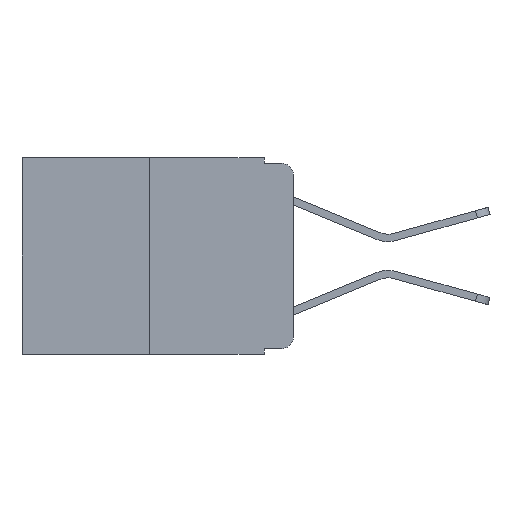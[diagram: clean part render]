
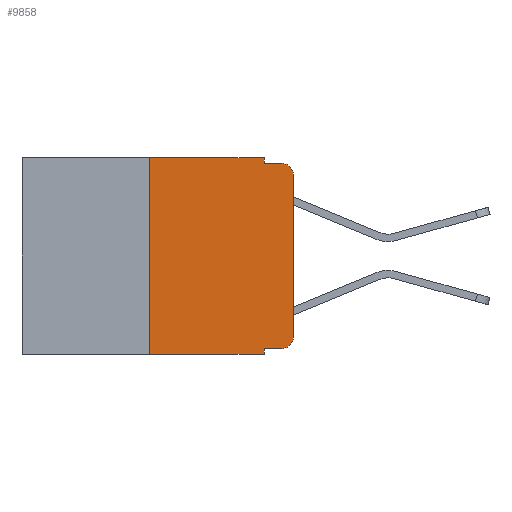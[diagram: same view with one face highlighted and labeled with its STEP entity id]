
A CAD part, left-side view. The second image highlights one B-rep face of the part: STEP entity #9858.
In plain terms, the highlighted planar face has unit normal (-1, 0, 0).
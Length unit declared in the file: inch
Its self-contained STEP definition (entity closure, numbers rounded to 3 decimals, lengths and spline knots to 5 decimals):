
#457 = CARTESIAN_POINT ( 'NONE',  ( 0., 0.25, 0. ) ) ;
#943 = EDGE_CURVE ( 'NONE', #7155, #8708, #5333, .T. ) ;
#949 = CARTESIAN_POINT ( 'NONE',  ( 0., 0.051, -0.333 ) ) ;
#1145 = ORIENTED_EDGE ( 'NONE', *, *, #11439, .T. ) ;
#1401 = DIRECTION ( 'NONE',  ( 0., 0., -1. ) ) ;
#1441 = ORIENTED_EDGE ( 'NONE', *, *, #943, .F. ) ;
#1490 = DIRECTION ( 'NONE',  ( 0., 0., 1. ) ) ;
#1531 = CARTESIAN_POINT ( 'NONE',  ( 0., 0.051, -0.333 ) ) ;
#1535 = PLANE ( 'NONE',  #4030 ) ;
#1721 = ORIENTED_EDGE ( 'NONE', *, *, #6857, .T. ) ;
#1846 = EDGE_CURVE ( 'NONE', #9617, #7839, #5854, .T. ) ;
#1906 = VECTOR ( 'NONE', #2562, 39.37008 ) ;
#1918 = CARTESIAN_POINT ( 'NONE',  ( 0., 0.02, -0.03 ) ) ;
#1947 = ORIENTED_EDGE ( 'NONE', *, *, #4604, .T. ) ;
#2239 = ORIENTED_EDGE ( 'NONE', *, *, #6475, .T. ) ;
#2348 = ORIENTED_EDGE ( 'NONE', *, *, #1846, .F. ) ;
#2426 = ORIENTED_EDGE ( 'NONE', *, *, #5461, .T. ) ;
#2505 = CARTESIAN_POINT ( 'NONE',  ( 0., 0.02, -0.313 ) ) ;
#2562 = DIRECTION ( 'NONE',  ( 0., -1., 0. ) ) ;
#2704 = VECTOR ( 'NONE', #1490, 39.37008 ) ;
#2751 = ORIENTED_EDGE ( 'NONE', *, *, #11470, .F. ) ;
#2771 = EDGE_CURVE ( 'NONE', #4984, #7155, #8645, .T. ) ;
#2778 = ORIENTED_EDGE ( 'NONE', *, *, #10975, .F. ) ;
#2969 = DIRECTION ( 'NONE',  ( 0., 0., -1. ) ) ;
#3091 = CARTESIAN_POINT ( 'NONE',  ( 0., 0.051, -0.01 ) ) ;
#3151 = CARTESIAN_POINT ( 'NONE',  ( 0., 0., -0.03 ) ) ;
#3328 = ORIENTED_EDGE ( 'NONE', *, *, #2771, .F. ) ;
#3361 = VECTOR ( 'NONE', #6061, 39.37008 ) ;
#3506 = CARTESIAN_POINT ( 'NONE',  ( 0., 0., 0. ) ) ;
#3539 = DIRECTION ( 'NONE',  ( 0., 0., -1. ) ) ;
#3949 = CARTESIAN_POINT ( 'NONE',  ( 0., 0.02, -0.333 ) ) ;
#4030 = AXIS2_PLACEMENT_3D ( 'NONE', #5511, #12036, #6426 ) ;
#4118 = DIRECTION ( 'NONE',  ( 0., -1., 0. ) ) ;
#4193 = VERTEX_POINT ( 'NONE', #4708 ) ;
#4548 = LINE ( 'NONE', #7319, #1906 ) ;
#4604 = EDGE_CURVE ( 'NONE', #4193, #6598, #8902, .T. ) ;
#4708 = CARTESIAN_POINT ( 'NONE',  ( 0., 0., -0.313 ) ) ;
#4772 = VERTEX_POINT ( 'NONE', #8410 ) ;
#4984 = VERTEX_POINT ( 'NONE', #6372 ) ;
#5025 = LINE ( 'NONE', #1531, #12170 ) ;
#5037 = VECTOR ( 'NONE', #8618, 39.37008 ) ;
#5267 = CIRCLE ( 'NONE', #10275, 0.02 ) ;
#5333 = LINE ( 'NONE', #7799, #5037 ) ;
#5461 = EDGE_CURVE ( 'NONE', #7344, #7839, #9170, .T. ) ;
#5469 = DIRECTION ( 'NONE',  ( 0., 0., 1. ) ) ;
#5511 = CARTESIAN_POINT ( 'NONE',  ( 0., 0.473, 0. ) ) ;
#5854 = LINE ( 'NONE', #6875, #3361 ) ;
#6061 = DIRECTION ( 'NONE',  ( 0., 0., -1. ) ) ;
#6119 = VECTOR ( 'NONE', #1401, 39.37008 ) ;
#6372 = CARTESIAN_POINT ( 'NONE',  ( 0., 0.051, 0. ) ) ;
#6403 = CARTESIAN_POINT ( 'NONE',  ( 0., 0.02, -0.01 ) ) ;
#6415 = DIRECTION ( 'NONE',  ( 0., -1., 0. ) ) ;
#6426 = DIRECTION ( 'NONE',  ( 0., 0., -1. ) ) ;
#6475 = EDGE_CURVE ( 'NONE', #6598, #8708, #7349, .T. ) ;
#6598 = VERTEX_POINT ( 'NONE', #3151 ) ;
#6857 = EDGE_CURVE ( 'NONE', #9617, #7717, #5025, .T. ) ;
#6875 = CARTESIAN_POINT ( 'NONE',  ( 0., 0.051, 0. ) ) ;
#7155 = VERTEX_POINT ( 'NONE', #3091 ) ;
#7319 = CARTESIAN_POINT ( 'NONE',  ( 0., 0.473, 0. ) ) ;
#7344 = VERTEX_POINT ( 'NONE', #9015 ) ;
#7349 = CIRCLE ( 'NONE', #8718, 0.02 ) ;
#7460 = LINE ( 'NONE', #457, #2704 ) ;
#7717 = VERTEX_POINT ( 'NONE', #3949 ) ;
#7799 = CARTESIAN_POINT ( 'NONE',  ( 0., 0.051, -0.01 ) ) ;
#7839 = VERTEX_POINT ( 'NONE', #11536 ) ;
#8410 = CARTESIAN_POINT ( 'NONE',  ( 0., 0.25, 0. ) ) ;
#8618 = DIRECTION ( 'NONE',  ( 0., -1., 0. ) ) ;
#8645 = LINE ( 'NONE', #10462, #6119 ) ;
#8652 = DIRECTION ( 'NONE',  ( -1., 0., 0. ) ) ;
#8663 = FACE_OUTER_BOUND ( 'NONE', #11680, .T. ) ;
#8708 = VERTEX_POINT ( 'NONE', #6403 ) ;
#8718 = AXIS2_PLACEMENT_3D ( 'NONE', #1918, #8652, #2969 ) ;
#8798 = CARTESIAN_POINT ( 'NONE',  ( 0., 0.473, -0.343 ) ) ;
#8881 = VECTOR ( 'NONE', #4118, 39.37008 ) ;
#8902 = LINE ( 'NONE', #3506, #10798 ) ;
#9015 = CARTESIAN_POINT ( 'NONE',  ( 0., 0.25, -0.343 ) ) ;
#9170 = LINE ( 'NONE', #8798, #8881 ) ;
#9186 = DIRECTION ( 'NONE',  ( -1., 0., 0. ) ) ;
#9617 = VERTEX_POINT ( 'NONE', #949 ) ;
#9858 = ADVANCED_FACE ( 'NONE', ( #8663 ), #1535, .F. ) ;
#10275 = AXIS2_PLACEMENT_3D ( 'NONE', #2505, #9186, #3539 ) ;
#10462 = CARTESIAN_POINT ( 'NONE',  ( 0., 0.051, 0. ) ) ;
#10798 = VECTOR ( 'NONE', #5469, 39.37008 ) ;
#10975 = EDGE_CURVE ( 'NONE', #4772, #4984, #4548, .T. ) ;
#11439 = EDGE_CURVE ( 'NONE', #7717, #4193, #5267, .T. ) ;
#11470 = EDGE_CURVE ( 'NONE', #7344, #4772, #7460, .T. ) ;
#11536 = CARTESIAN_POINT ( 'NONE',  ( 0., 0.051, -0.343 ) ) ;
#11680 = EDGE_LOOP ( 'NONE', ( #1947, #2239, #1441, #3328, #2778, #2751, #2426, #2348, #1721, #1145 ) ) ;
#12036 = DIRECTION ( 'NONE',  ( 1., 0., 0. ) ) ;
#12170 = VECTOR ( 'NONE', #6415, 39.37008 ) ;
